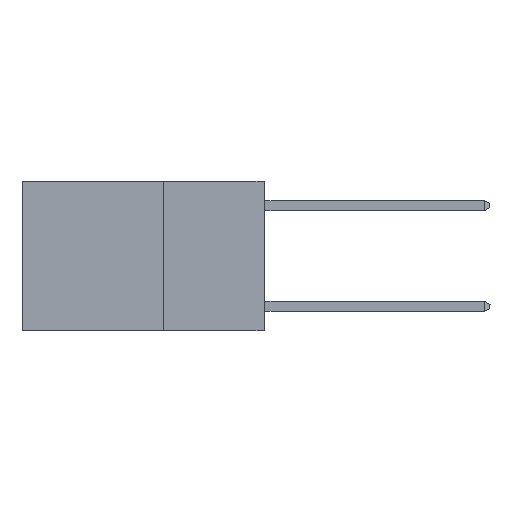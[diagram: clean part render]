
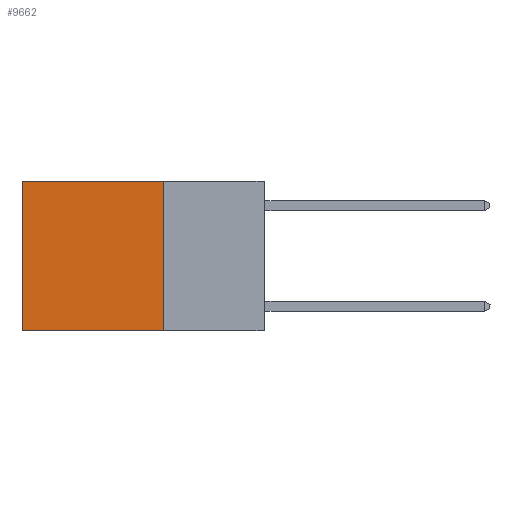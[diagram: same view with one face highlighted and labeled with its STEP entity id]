
A CAD part, left-side view. The second image highlights one B-rep face of the part: STEP entity #9662.
In plain terms, the highlighted planar face has unit normal (-1, 0, 0).
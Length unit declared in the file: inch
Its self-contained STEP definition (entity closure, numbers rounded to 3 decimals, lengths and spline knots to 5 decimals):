
#213 = CARTESIAN_POINT ( 'NONE',  ( 0.2625, 0.25, 0. ) ) ;
#503 = CARTESIAN_POINT ( 'NONE',  ( 0.2625, 0.25, -0.37 ) ) ;
#683 = VECTOR ( 'NONE', #6950, 39.37008 ) ;
#816 = VERTEX_POINT ( 'NONE', #503 ) ;
#1146 = LINE ( 'NONE', #16985, #683 ) ;
#1201 = EDGE_CURVE ( 'NONE', #10398, #5703, #1146, .T. ) ;
#1681 = DIRECTION ( 'NONE',  ( 0., 0., -1. ) ) ;
#1881 = ORIENTED_EDGE ( 'NONE', *, *, #1201, .T. ) ;
#1925 = DIRECTION ( 'NONE',  ( 0., 1., 0. ) ) ;
#2081 = VERTEX_POINT ( 'NONE', #213 ) ;
#3096 = EDGE_LOOP ( 'NONE', ( #1881, #7913, #14926, #13381 ) ) ;
#3118 = CARTESIAN_POINT ( 'NONE',  ( 0.2625, 0.25, 0. ) ) ;
#3784 = EDGE_CURVE ( 'NONE', #2081, #816, #4010, .T. ) ;
#4010 = LINE ( 'NONE', #3118, #10339 ) ;
#4493 = CARTESIAN_POINT ( 'NONE',  ( 0.2625, 0.6, -0.37 ) ) ;
#5703 = VERTEX_POINT ( 'NONE', #4493 ) ;
#5765 = AXIS2_PLACEMENT_3D ( 'NONE', #10224, #6252, #15624 ) ;
#6252 = DIRECTION ( 'NONE',  ( 1., 0., 0. ) ) ;
#6950 = DIRECTION ( 'NONE',  ( 0., 0., -1. ) ) ;
#7081 = VECTOR ( 'NONE', #1925, 39.37008 ) ;
#7289 = DIRECTION ( 'NONE',  ( 0., 1., 0. ) ) ;
#7494 = VECTOR ( 'NONE', #7289, 39.37008 ) ;
#7652 = FACE_OUTER_BOUND ( 'NONE', #3096, .T. ) ;
#7910 = LINE ( 'NONE', #14000, #7494 ) ;
#7913 = ORIENTED_EDGE ( 'NONE', *, *, #8399, .F. ) ;
#8399 = EDGE_CURVE ( 'NONE', #816, #5703, #7910, .T. ) ;
#8424 = EDGE_CURVE ( 'NONE', #2081, #10398, #10615, .T. ) ;
#9662 = ADVANCED_FACE ( 'NONE', ( #7652 ), #12911, .F. ) ;
#10224 = CARTESIAN_POINT ( 'NONE',  ( 0.2625, 0.25, 0. ) ) ;
#10339 = VECTOR ( 'NONE', #1681, 39.37008 ) ;
#10398 = VERTEX_POINT ( 'NONE', #11720 ) ;
#10615 = LINE ( 'NONE', #14053, #7081 ) ;
#11720 = CARTESIAN_POINT ( 'NONE',  ( 0.2625, 0.6, 0. ) ) ;
#12911 = PLANE ( 'NONE',  #5765 ) ;
#13381 = ORIENTED_EDGE ( 'NONE', *, *, #8424, .T. ) ;
#14000 = CARTESIAN_POINT ( 'NONE',  ( 0.2625, 0.25, -0.37 ) ) ;
#14053 = CARTESIAN_POINT ( 'NONE',  ( 0.2625, 0.25, 0. ) ) ;
#14926 = ORIENTED_EDGE ( 'NONE', *, *, #3784, .F. ) ;
#15624 = DIRECTION ( 'NONE',  ( 0., 0., -1. ) ) ;
#16985 = CARTESIAN_POINT ( 'NONE',  ( 0.2625, 0.6, 0. ) ) ;
